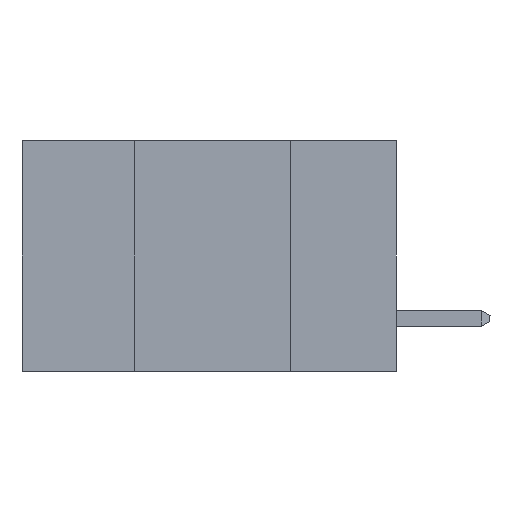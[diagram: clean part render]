
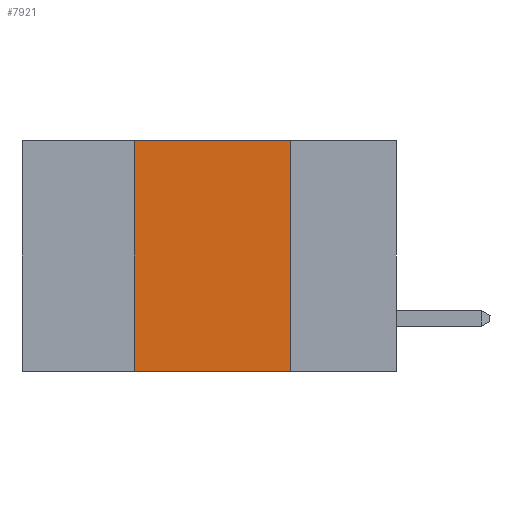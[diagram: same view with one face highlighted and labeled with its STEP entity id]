
A CAD part, left-side view. The second image highlights one B-rep face of the part: STEP entity #7921.
In plain terms, the highlighted planar face has unit normal (-1, 0, 0).
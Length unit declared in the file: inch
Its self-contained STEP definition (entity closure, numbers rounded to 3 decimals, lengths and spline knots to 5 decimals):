
#2 = VECTOR ( 'NONE', #16887, 39.37008 ) ;
#456 = DIRECTION ( 'NONE',  ( 0., -1., 0. ) ) ;
#560 = CARTESIAN_POINT ( 'NONE',  ( 0., 0.6, 0. ) ) ;
#1064 = ORIENTED_EDGE ( 'NONE', *, *, #5846, .F. ) ;
#1242 = VERTEX_POINT ( 'NONE', #16219 ) ;
#1694 = LINE ( 'NONE', #4118, #10093 ) ;
#2196 = FACE_OUTER_BOUND ( 'NONE', #16721, .T. ) ;
#2389 = VECTOR ( 'NONE', #13590, 39.37008 ) ;
#2488 = ORIENTED_EDGE ( 'NONE', *, *, #11932, .T. ) ;
#4118 = CARTESIAN_POINT ( 'NONE',  ( 0., 0.6, -0.37 ) ) ;
#4507 = AXIS2_PLACEMENT_3D ( 'NONE', #8056, #8051, #8035 ) ;
#4844 = CARTESIAN_POINT ( 'NONE',  ( 0., 0.17, 0. ) ) ;
#5781 = LINE ( 'NONE', #560, #13219 ) ;
#5846 = EDGE_CURVE ( 'NONE', #1242, #9770, #5781, .T. ) ;
#6342 = VERTEX_POINT ( 'NONE', #7158 ) ;
#7158 = CARTESIAN_POINT ( 'NONE',  ( 0., 0.42, -0.37 ) ) ;
#7860 = ORIENTED_EDGE ( 'NONE', *, *, #9118, .F. ) ;
#7875 = CARTESIAN_POINT ( 'NONE',  ( 0., 0.42, -0.37 ) ) ;
#7921 = ADVANCED_FACE ( 'NONE', ( #2196 ), #8093, .F. ) ;
#8035 = DIRECTION ( 'NONE',  ( 0., 0., -1. ) ) ;
#8051 = DIRECTION ( 'NONE',  ( 1., 0., 0. ) ) ;
#8056 = CARTESIAN_POINT ( 'NONE',  ( 0., 0.6, 0. ) ) ;
#8093 = PLANE ( 'NONE',  #4507 ) ;
#8590 = ORIENTED_EDGE ( 'NONE', *, *, #9001, .F. ) ;
#9001 = EDGE_CURVE ( 'NONE', #9770, #15429, #10313, .T. ) ;
#9118 = EDGE_CURVE ( 'NONE', #6342, #1242, #11913, .T. ) ;
#9386 = CARTESIAN_POINT ( 'NONE',  ( 0., 0.17, -0.37 ) ) ;
#9770 = VERTEX_POINT ( 'NONE', #4844 ) ;
#10093 = VECTOR ( 'NONE', #10110, 39.37008 ) ;
#10110 = DIRECTION ( 'NONE',  ( 0., -1., 0. ) ) ;
#10313 = LINE ( 'NONE', #12086, #2389 ) ;
#11913 = LINE ( 'NONE', #7875, #2 ) ;
#11932 = EDGE_CURVE ( 'NONE', #6342, #15429, #1694, .T. ) ;
#12086 = CARTESIAN_POINT ( 'NONE',  ( 0., 0.17, -0.37 ) ) ;
#13219 = VECTOR ( 'NONE', #456, 39.37008 ) ;
#13590 = DIRECTION ( 'NONE',  ( 0., 0., -1. ) ) ;
#15429 = VERTEX_POINT ( 'NONE', #9386 ) ;
#16219 = CARTESIAN_POINT ( 'NONE',  ( 0., 0.42, 0. ) ) ;
#16721 = EDGE_LOOP ( 'NONE', ( #8590, #1064, #7860, #2488 ) ) ;
#16887 = DIRECTION ( 'NONE',  ( 0., 0., 1. ) ) ;
